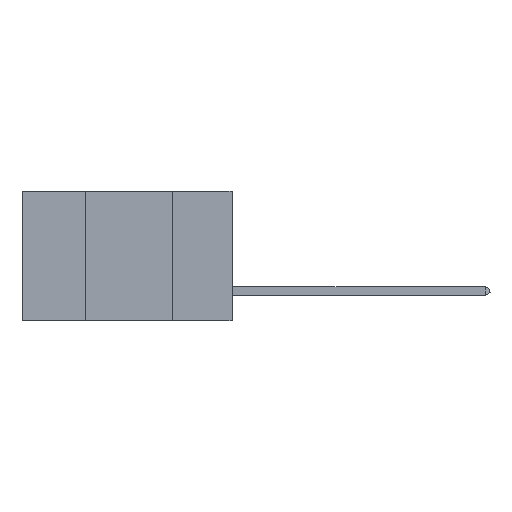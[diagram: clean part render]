
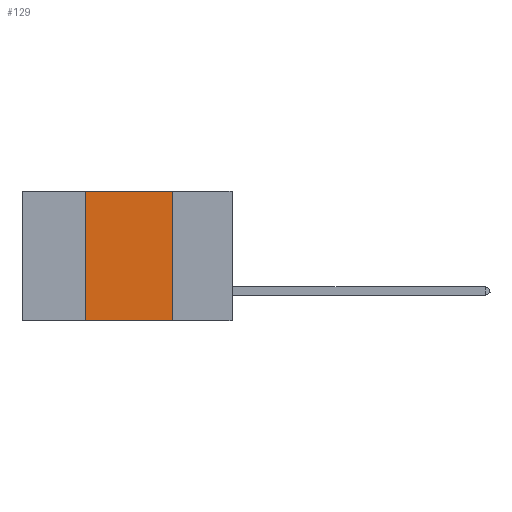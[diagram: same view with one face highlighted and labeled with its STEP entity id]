
A CAD part, left-side view. The second image highlights one B-rep face of the part: STEP entity #129.
In plain terms, the highlighted planar face has unit normal (-1, 0, 0).
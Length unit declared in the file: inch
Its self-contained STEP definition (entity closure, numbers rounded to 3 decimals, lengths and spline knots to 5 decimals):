
#53 = EDGE_LOOP ( 'NONE', ( #10190, #5959, #8787, #752 ) ) ;
#129 = ADVANCED_FACE ( 'NONE', ( #10553 ), #2431, .F. ) ;
#262 = DIRECTION ( 'NONE',  ( 0., 0., 1. ) ) ;
#295 = CARTESIAN_POINT ( 'NONE',  ( 0., 0.42, 0. ) ) ;
#447 = DIRECTION ( 'NONE',  ( 0., 0., -1. ) ) ;
#752 = ORIENTED_EDGE ( 'NONE', *, *, #6229, .T. ) ;
#777 = EDGE_CURVE ( 'NONE', #8580, #8261, #4298, .T. ) ;
#1215 = CARTESIAN_POINT ( 'NONE',  ( 0., 0.42, 0. ) ) ;
#2431 = PLANE ( 'NONE',  #4050 ) ;
#2710 = CARTESIAN_POINT ( 'NONE',  ( 0., 0.17, 0. ) ) ;
#2890 = CARTESIAN_POINT ( 'NONE',  ( 0., 0.6, -0.37 ) ) ;
#3135 = EDGE_CURVE ( 'NONE', #8261, #10603, #6385, .T. ) ;
#3477 = CARTESIAN_POINT ( 'NONE',  ( 0., 0.17, 0. ) ) ;
#4050 = AXIS2_PLACEMENT_3D ( 'NONE', #12451, #9293, #10308 ) ;
#4274 = DIRECTION ( 'NONE',  ( 0., -1., 0. ) ) ;
#4298 = LINE ( 'NONE', #10134, #9434 ) ;
#4596 = VECTOR ( 'NONE', #4921, 39.37008 ) ;
#4921 = DIRECTION ( 'NONE',  ( 0., -1., 0. ) ) ;
#5484 = VERTEX_POINT ( 'NONE', #11794 ) ;
#5959 = ORIENTED_EDGE ( 'NONE', *, *, #777, .F. ) ;
#6229 = EDGE_CURVE ( 'NONE', #5484, #10603, #7263, .T. ) ;
#6385 = LINE ( 'NONE', #3477, #10773 ) ;
#7263 = LINE ( 'NONE', #2890, #4596 ) ;
#7606 = CARTESIAN_POINT ( 'NONE',  ( 0., 0.17, -0.37 ) ) ;
#7810 = EDGE_CURVE ( 'NONE', #5484, #8580, #9642, .T. ) ;
#8261 = VERTEX_POINT ( 'NONE', #2710 ) ;
#8580 = VERTEX_POINT ( 'NONE', #295 ) ;
#8787 = ORIENTED_EDGE ( 'NONE', *, *, #7810, .F. ) ;
#9293 = DIRECTION ( 'NONE',  ( 1., 0., 0. ) ) ;
#9434 = VECTOR ( 'NONE', #4274, 39.37008 ) ;
#9642 = LINE ( 'NONE', #1215, #12780 ) ;
#10134 = CARTESIAN_POINT ( 'NONE',  ( 0., 0.6, 0. ) ) ;
#10190 = ORIENTED_EDGE ( 'NONE', *, *, #3135, .F. ) ;
#10308 = DIRECTION ( 'NONE',  ( 0., 0., -1. ) ) ;
#10553 = FACE_OUTER_BOUND ( 'NONE', #53, .T. ) ;
#10603 = VERTEX_POINT ( 'NONE', #7606 ) ;
#10773 = VECTOR ( 'NONE', #447, 39.37008 ) ;
#11794 = CARTESIAN_POINT ( 'NONE',  ( 0., 0.42, -0.37 ) ) ;
#12451 = CARTESIAN_POINT ( 'NONE',  ( 0., 0.6, 0. ) ) ;
#12780 = VECTOR ( 'NONE', #262, 39.37008 ) ;
